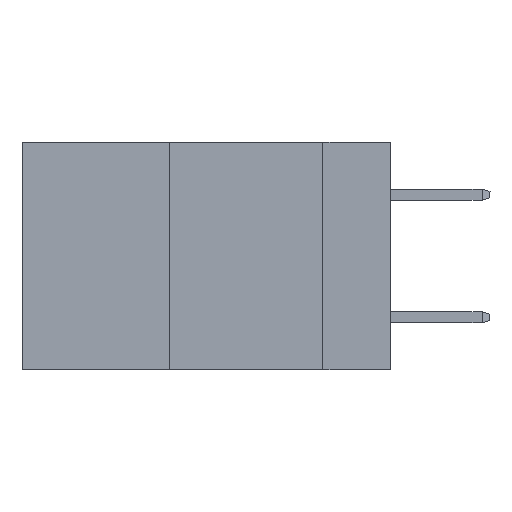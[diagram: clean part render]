
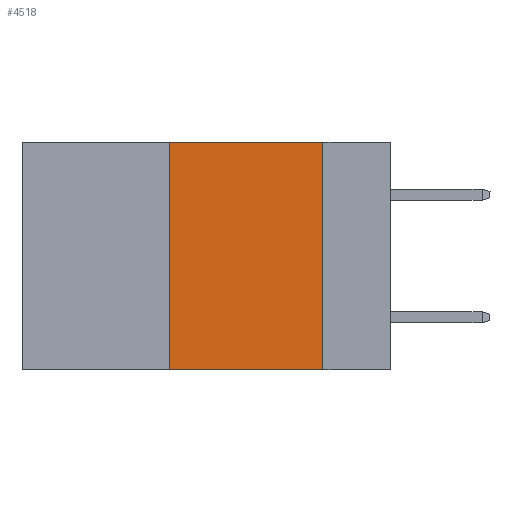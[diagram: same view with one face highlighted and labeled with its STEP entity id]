
A CAD part, left-side view. The second image highlights one B-rep face of the part: STEP entity #4518.
In plain terms, the highlighted planar face has unit normal (-1, 0, 0).
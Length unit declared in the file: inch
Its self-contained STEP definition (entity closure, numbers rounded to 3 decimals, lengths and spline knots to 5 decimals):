
#389 = DIRECTION ( 'NONE',  ( 0., -1., 0. ) ) ;
#568 = EDGE_CURVE ( 'NONE', #5553, #10076, #7696, .T. ) ;
#1031 = DIRECTION ( 'NONE',  ( 0., 0., -1. ) ) ;
#1123 = VECTOR ( 'NONE', #389, 39.37008 ) ;
#1218 = EDGE_CURVE ( 'NONE', #5553, #6572, #8650, .T. ) ;
#1345 = CARTESIAN_POINT ( 'NONE',  ( 0., 0.6, 0. ) ) ;
#1632 = DIRECTION ( 'NONE',  ( 0., -1., 0. ) ) ;
#1667 = CARTESIAN_POINT ( 'NONE',  ( 0., 0.36, 0. ) ) ;
#1824 = EDGE_CURVE ( 'NONE', #6879, #10076, #9319, .T. ) ;
#2145 = EDGE_CURVE ( 'NONE', #6572, #6879, #3587, .T. ) ;
#2432 = VECTOR ( 'NONE', #2770, 39.37008 ) ;
#2729 = CARTESIAN_POINT ( 'NONE',  ( 0., 0.11, 0. ) ) ;
#2770 = DIRECTION ( 'NONE',  ( 0., 0., -1. ) ) ;
#3021 = ORIENTED_EDGE ( 'NONE', *, *, #1824, .F. ) ;
#3046 = CARTESIAN_POINT ( 'NONE',  ( 0., 0.11, 0. ) ) ;
#3510 = CARTESIAN_POINT ( 'NONE',  ( 0., 0.11, -0.37 ) ) ;
#3570 = EDGE_LOOP ( 'NONE', ( #3021, #5415, #7805, #5690 ) ) ;
#3587 = LINE ( 'NONE', #1345, #1123 ) ;
#3638 = DIRECTION ( 'NONE',  ( 0., 0., 1. ) ) ;
#4518 = ADVANCED_FACE ( 'NONE', ( #7320 ), #10866, .F. ) ;
#5415 = ORIENTED_EDGE ( 'NONE', *, *, #2145, .F. ) ;
#5553 = VERTEX_POINT ( 'NONE', #8251 ) ;
#5595 = CARTESIAN_POINT ( 'NONE',  ( 0., 0.6, 0. ) ) ;
#5690 = ORIENTED_EDGE ( 'NONE', *, *, #568, .T. ) ;
#5713 = CARTESIAN_POINT ( 'NONE',  ( 0., 0.6, -0.37 ) ) ;
#6267 = VECTOR ( 'NONE', #3638, 39.37008 ) ;
#6469 = DIRECTION ( 'NONE',  ( 1., 0., 0. ) ) ;
#6572 = VERTEX_POINT ( 'NONE', #10629 ) ;
#6879 = VERTEX_POINT ( 'NONE', #3046 ) ;
#7320 = FACE_OUTER_BOUND ( 'NONE', #3570, .T. ) ;
#7696 = LINE ( 'NONE', #5713, #7982 ) ;
#7805 = ORIENTED_EDGE ( 'NONE', *, *, #1218, .F. ) ;
#7982 = VECTOR ( 'NONE', #1632, 39.37008 ) ;
#8251 = CARTESIAN_POINT ( 'NONE',  ( 0., 0.36, -0.37 ) ) ;
#8650 = LINE ( 'NONE', #1667, #6267 ) ;
#9319 = LINE ( 'NONE', #2729, #2432 ) ;
#9658 = AXIS2_PLACEMENT_3D ( 'NONE', #5595, #6469, #1031 ) ;
#10076 = VERTEX_POINT ( 'NONE', #3510 ) ;
#10629 = CARTESIAN_POINT ( 'NONE',  ( 0., 0.36, 0. ) ) ;
#10866 = PLANE ( 'NONE',  #9658 ) ;
